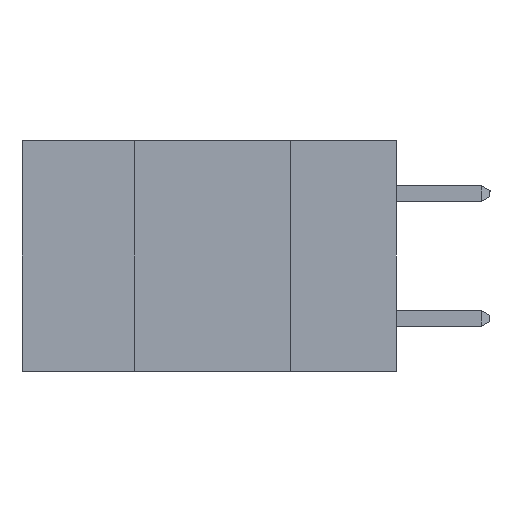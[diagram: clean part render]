
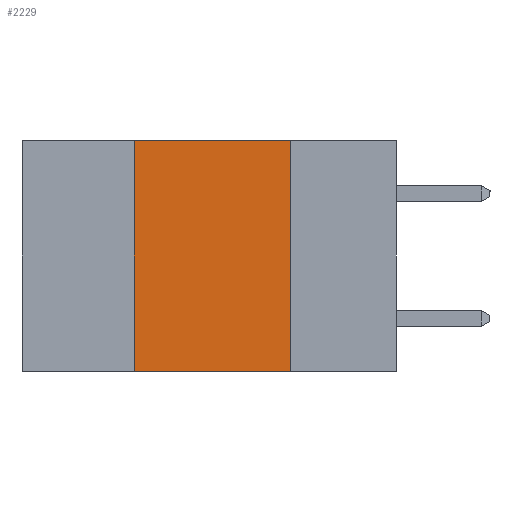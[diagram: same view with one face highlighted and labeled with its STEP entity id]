
A CAD part, left-side view. The second image highlights one B-rep face of the part: STEP entity #2229.
In plain terms, the highlighted planar face has unit normal (-1, 0, 0).
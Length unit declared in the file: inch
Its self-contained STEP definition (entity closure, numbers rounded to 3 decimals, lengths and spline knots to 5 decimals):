
#465 = DIRECTION ( 'NONE',  ( 1., 0., 0. ) ) ;
#763 = EDGE_CURVE ( 'NONE', #18119, #10960, #7790, .T. ) ;
#1655 = VECTOR ( 'NONE', #14128, 39.37008 ) ;
#1746 = VECTOR ( 'NONE', #6191, 39.37008 ) ;
#1978 = CARTESIAN_POINT ( 'NONE',  ( 0., 0.6, 0. ) ) ;
#2229 = ADVANCED_FACE ( 'NONE', ( #25054 ), #2515, .F. ) ;
#2238 = DIRECTION ( 'NONE',  ( 0., -1., 0. ) ) ;
#2515 = PLANE ( 'NONE',  #5656 ) ;
#2553 = CARTESIAN_POINT ( 'NONE',  ( 0., 0.17, -0.37 ) ) ;
#2641 = LINE ( 'NONE', #14654, #22530 ) ;
#4926 = EDGE_CURVE ( 'NONE', #10960, #18894, #13085, .T. ) ;
#5532 = CARTESIAN_POINT ( 'NONE',  ( 0., 0.17, 0. ) ) ;
#5599 = CARTESIAN_POINT ( 'NONE',  ( 0., 0.42, 0. ) ) ;
#5656 = AXIS2_PLACEMENT_3D ( 'NONE', #1978, #465, #8718 ) ;
#6084 = ORIENTED_EDGE ( 'NONE', *, *, #15788, .F. ) ;
#6191 = DIRECTION ( 'NONE',  ( 0., 0., 1. ) ) ;
#7702 = CARTESIAN_POINT ( 'NONE',  ( 0., 0.42, -0.37 ) ) ;
#7790 = LINE ( 'NONE', #10204, #1655 ) ;
#8718 = DIRECTION ( 'NONE',  ( 0., 0., -1. ) ) ;
#9754 = EDGE_LOOP ( 'NONE', ( #17271, #12434, #6084, #10720 ) ) ;
#10204 = CARTESIAN_POINT ( 'NONE',  ( 0., 0.6, 0. ) ) ;
#10720 = ORIENTED_EDGE ( 'NONE', *, *, #16369, .T. ) ;
#10960 = VERTEX_POINT ( 'NONE', #5532 ) ;
#12434 = ORIENTED_EDGE ( 'NONE', *, *, #763, .F. ) ;
#12815 = DIRECTION ( 'NONE',  ( 0., 0., -1. ) ) ;
#13085 = LINE ( 'NONE', #2553, #14750 ) ;
#14128 = DIRECTION ( 'NONE',  ( 0., -1., 0. ) ) ;
#14654 = CARTESIAN_POINT ( 'NONE',  ( 0., 0.6, -0.37 ) ) ;
#14750 = VECTOR ( 'NONE', #12815, 39.37008 ) ;
#15023 = VERTEX_POINT ( 'NONE', #20831 ) ;
#15788 = EDGE_CURVE ( 'NONE', #15023, #18119, #24283, .T. ) ;
#16369 = EDGE_CURVE ( 'NONE', #15023, #18894, #2641, .T. ) ;
#17271 = ORIENTED_EDGE ( 'NONE', *, *, #4926, .F. ) ;
#18119 = VERTEX_POINT ( 'NONE', #5599 ) ;
#18894 = VERTEX_POINT ( 'NONE', #26221 ) ;
#20831 = CARTESIAN_POINT ( 'NONE',  ( 0., 0.42, -0.37 ) ) ;
#22530 = VECTOR ( 'NONE', #2238, 39.37008 ) ;
#24283 = LINE ( 'NONE', #7702, #1746 ) ;
#25054 = FACE_OUTER_BOUND ( 'NONE', #9754, .T. ) ;
#26221 = CARTESIAN_POINT ( 'NONE',  ( 0., 0.17, -0.37 ) ) ;
